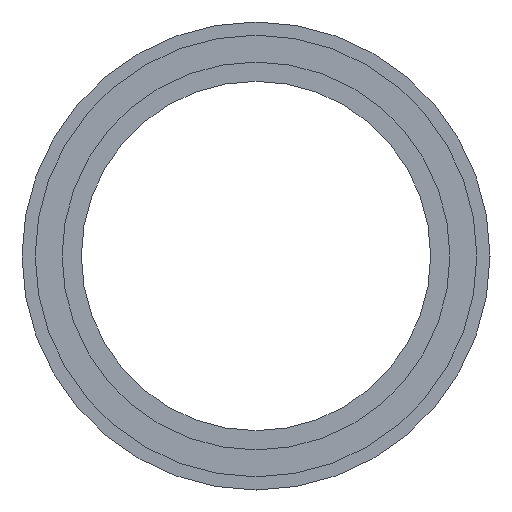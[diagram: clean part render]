
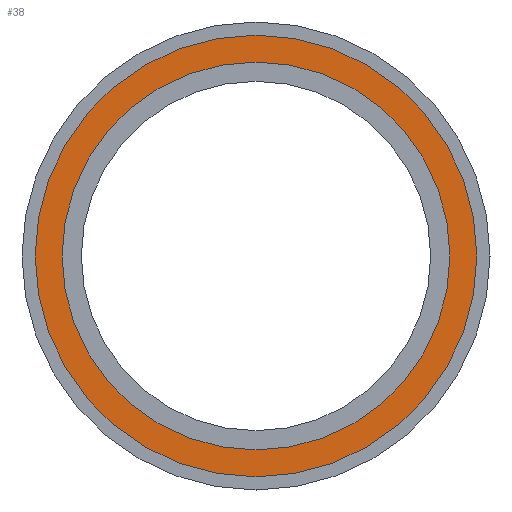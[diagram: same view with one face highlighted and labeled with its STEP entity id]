
A CAD part, front view. The second image highlights one B-rep face of the part: STEP entity #38.
In plain terms, the highlighted planar face has unit normal (0, -1, 0).
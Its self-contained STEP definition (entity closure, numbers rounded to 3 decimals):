
#13 = PLANE ( 'NONE',  #375 ) ;
#21 = CIRCLE ( 'NONE', #156, 35.3 ) ;
#30 = ORIENTED_EDGE ( 'NONE', *, *, #129, .T. ) ;
#37 = VERTEX_POINT ( 'NONE', #146 ) ;
#38 = ADVANCED_FACE ( 'NONE', ( #118, #219 ), #13, .F. ) ;
#60 = CARTESIAN_POINT ( 'NONE',  ( 0., 0., 0. ) ) ;
#73 = AXIS2_PLACEMENT_3D ( 'NONE', #387, #425, #354 ) ;
#76 = CARTESIAN_POINT ( 'NONE',  ( 0., 0., -40.2 ) ) ;
#86 = CARTESIAN_POINT ( 'NONE',  ( -35.3, 0., 0. ) ) ;
#93 = DIRECTION ( 'NONE',  ( 0., -1., 0. ) ) ;
#104 = EDGE_LOOP ( 'NONE', ( #161, #426 ) ) ;
#117 = DIRECTION ( 'NONE',  ( 0., 0., -1. ) ) ;
#118 = FACE_BOUND ( 'NONE', #104, .T. ) ;
#119 = CIRCLE ( 'NONE', #331, 40.2 ) ;
#120 = CARTESIAN_POINT ( 'NONE',  ( 0., 0., 0. ) ) ;
#129 = EDGE_CURVE ( 'NONE', #139, #332, #119, .T. ) ;
#139 = VERTEX_POINT ( 'NONE', #181 ) ;
#146 = CARTESIAN_POINT ( 'NONE',  ( 0., 0., -35.3 ) ) ;
#156 = AXIS2_PLACEMENT_3D ( 'NONE', #60, #93, #415 ) ;
#161 = ORIENTED_EDGE ( 'NONE', *, *, #362, .F. ) ;
#163 = DIRECTION ( 'NONE',  ( 0., 0., -1. ) ) ;
#181 = CARTESIAN_POINT ( 'NONE',  ( 0., 0., 40.2 ) ) ;
#183 = DIRECTION ( 'NONE',  ( 0., -1., 0. ) ) ;
#204 = EDGE_CURVE ( 'NONE', #423, #37, #21, .T. ) ;
#206 = CARTESIAN_POINT ( 'NONE',  ( 0., 0., 0. ) ) ;
#219 = FACE_OUTER_BOUND ( 'NONE', #263, .T. ) ;
#232 = DIRECTION ( 'NONE',  ( 0., -1., 0. ) ) ;
#243 = ORIENTED_EDGE ( 'NONE', *, *, #399, .T. ) ;
#249 = DIRECTION ( 'NONE',  ( 0., 1., 0. ) ) ;
#260 = AXIS2_PLACEMENT_3D ( 'NONE', #206, #232, #163 ) ;
#263 = EDGE_LOOP ( 'NONE', ( #243, #30 ) ) ;
#278 = CIRCLE ( 'NONE', #260, 40.2 ) ;
#306 = CIRCLE ( 'NONE', #73, 35.3 ) ;
#331 = AXIS2_PLACEMENT_3D ( 'NONE', #120, #183, #117 ) ;
#332 = VERTEX_POINT ( 'NONE', #76 ) ;
#354 = DIRECTION ( 'NONE',  ( 0., 0., -1. ) ) ;
#362 = EDGE_CURVE ( 'NONE', #37, #423, #306, .T. ) ;
#372 = CARTESIAN_POINT ( 'NONE',  ( 0., 0., 35.3 ) ) ;
#375 = AXIS2_PLACEMENT_3D ( 'NONE', #86, #249, #398 ) ;
#387 = CARTESIAN_POINT ( 'NONE',  ( 0., 0., 0. ) ) ;
#398 = DIRECTION ( 'NONE',  ( 0., 0., 1. ) ) ;
#399 = EDGE_CURVE ( 'NONE', #332, #139, #278, .T. ) ;
#415 = DIRECTION ( 'NONE',  ( 0., 0., -1. ) ) ;
#423 = VERTEX_POINT ( 'NONE', #372 ) ;
#425 = DIRECTION ( 'NONE',  ( 0., -1., 0. ) ) ;
#426 = ORIENTED_EDGE ( 'NONE', *, *, #204, .F. ) ;
